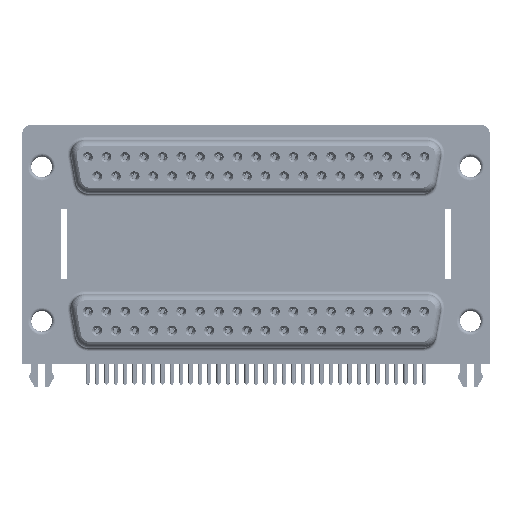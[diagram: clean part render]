
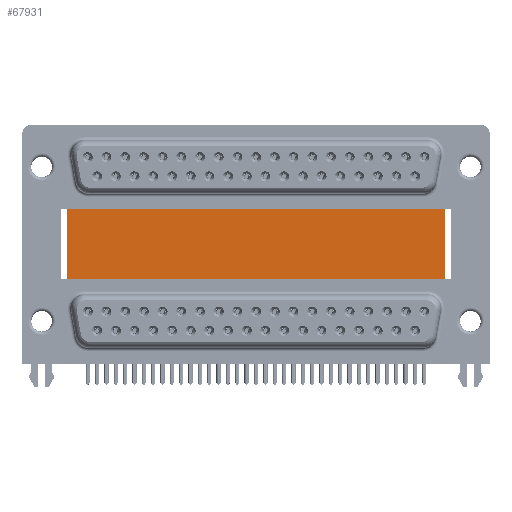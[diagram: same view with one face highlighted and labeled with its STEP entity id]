
A CAD part, top view. The second image highlights one B-rep face of the part: STEP entity #67931.
In plain terms, the highlighted planar face has unit normal (0, 0, 1).
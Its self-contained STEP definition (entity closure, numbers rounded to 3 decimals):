
#1650 = VECTOR ( 'NONE', #2195, 1000. ) ;
#2195 = DIRECTION ( 'NONE',  ( 1., 0., 0. ) ) ;
#3051 = ORIENTED_EDGE ( 'NONE', *, *, #29950, .T. ) ;
#3686 = LINE ( 'NONE', #26757, #25564 ) ;
#7753 = CARTESIAN_POINT ( 'NONE',  ( 3.79, -3.735, -12. ) ) ;
#8186 = VERTEX_POINT ( 'NONE', #7753 ) ;
#10827 = EDGE_CURVE ( 'NONE', #27736, #58902, #3686, .T. ) ;
#13424 = CARTESIAN_POINT ( 'NONE',  ( 59.71, 16.585, -12. ) ) ;
#14375 = CARTESIAN_POINT ( 'NONE',  ( 3.79, 16.585, -12. ) ) ;
#14767 = EDGE_CURVE ( 'NONE', #32159, #27736, #26768, .T. ) ;
#15445 = ORIENTED_EDGE ( 'NONE', *, *, #65907, .T. ) ;
#22079 = DIRECTION ( 'NONE',  ( 1., 0., 0. ) ) ;
#25564 = VECTOR ( 'NONE', #49774, 1000. ) ;
#26757 = CARTESIAN_POINT ( 'NONE',  ( 59.71, 16.585, -12. ) ) ;
#26768 = LINE ( 'NONE', #66747, #1650 ) ;
#27736 = VERTEX_POINT ( 'NONE', #13424 ) ;
#29382 = CARTESIAN_POINT ( 'NONE',  ( 3.79, 16.585, -12. ) ) ;
#29896 = DIRECTION ( 'NONE',  ( -1., 0., 0. ) ) ;
#29950 = EDGE_CURVE ( 'NONE', #32159, #8186, #64066, .T. ) ;
#30427 = VECTOR ( 'NONE', #68997, 1000. ) ;
#32159 = VERTEX_POINT ( 'NONE', #38222 ) ;
#36063 = ORIENTED_EDGE ( 'NONE', *, *, #10827, .F. ) ;
#37393 = DIRECTION ( 'NONE',  ( 0., 0., -1. ) ) ;
#37437 = CARTESIAN_POINT ( 'NONE',  ( 59.71, -3.735, -12. ) ) ;
#38222 = CARTESIAN_POINT ( 'NONE',  ( 3.79, 16.585, -12. ) ) ;
#42229 = ORIENTED_EDGE ( 'NONE', *, *, #14767, .F. ) ;
#43057 = FACE_OUTER_BOUND ( 'NONE', #48126, .T. ) ;
#45445 = CARTESIAN_POINT ( 'NONE',  ( 3.79, -3.735, -12. ) ) ;
#47630 = PLANE ( 'NONE',  #54296 ) ;
#48126 = EDGE_LOOP ( 'NONE', ( #15445, #36063, #42229, #3051 ) ) ;
#49774 = DIRECTION ( 'NONE',  ( 0., -1., 0. ) ) ;
#54296 = AXIS2_PLACEMENT_3D ( 'NONE', #14375, #37393, #29896 ) ;
#58902 = VERTEX_POINT ( 'NONE', #37437 ) ;
#64066 = LINE ( 'NONE', #29382, #30427 ) ;
#65907 = EDGE_CURVE ( 'NONE', #8186, #58902, #74140, .T. ) ;
#66747 = CARTESIAN_POINT ( 'NONE',  ( 3.79, 16.585, -12. ) ) ;
#67931 = ADVANCED_FACE ( 'NONE', ( #43057 ), #47630, .F. ) ;
#68997 = DIRECTION ( 'NONE',  ( 0., -1., 0. ) ) ;
#73312 = VECTOR ( 'NONE', #22079, 1000. ) ;
#74140 = LINE ( 'NONE', #45445, #73312 ) ;
